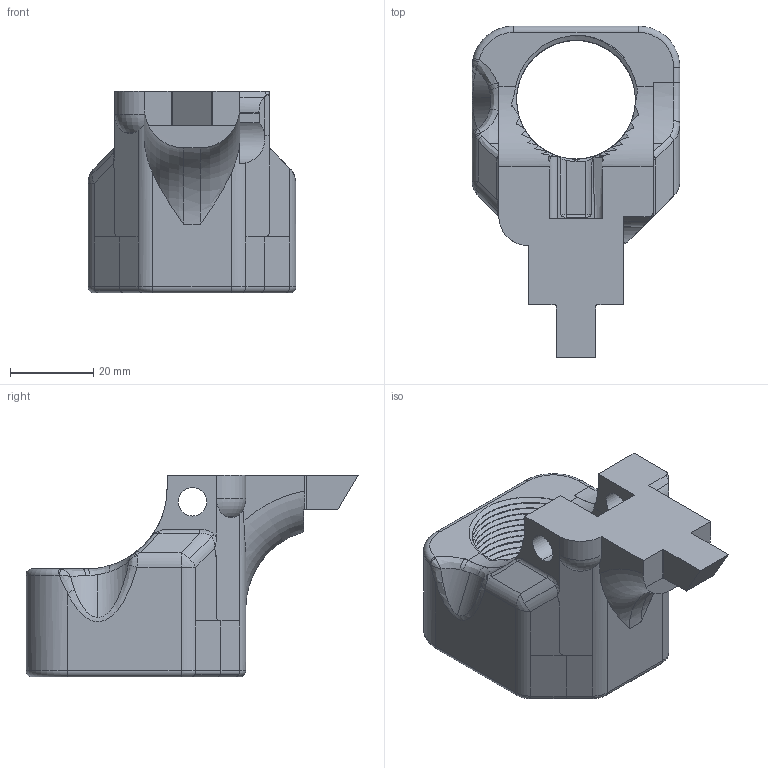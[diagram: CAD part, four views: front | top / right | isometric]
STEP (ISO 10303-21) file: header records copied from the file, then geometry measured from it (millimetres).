
FILE_DESCRIPTION (( 'STEP AP214' ), '1' );
FILE_NAME ('Hermes_V1.4_Rear.STEP', '2015-05-21T07:12:21', ( 'WarFairy' ), ( '' ), 'SwSTEP 2.0', 'SolidWorks 2015', '' );
FILE_SCHEMA (( 'AUTOMOTIVE_DESIGN' ));
Length unit declared in the file: inch
Products named in the file (1): Hermes_V1.4_Rear
Bounding box: 50 x 79.86 x 48.55 mm (x, y, z)
Volume: 64253.8 mm3; surface area: 17497.2 mm2
Topology: 1 solids, 1 shells, 223 faces, 669 edges, 443 vertices
Faces by surface type: cylinder 102, bspline 53, plane 49, torus 15, cone 3, sphere 1
Entity records: 21281 total; most frequent: CARTESIAN_POINT 16105, ORIENTED_EDGE 1330, DIRECTION 748, EDGE_CURVE 665, VERTEX_POINT 443, B_SPLINE_CURVE_WITH_KNOTS 311, AXIS2_PLACEMENT_3D 284, EDGE_LOOP 228
